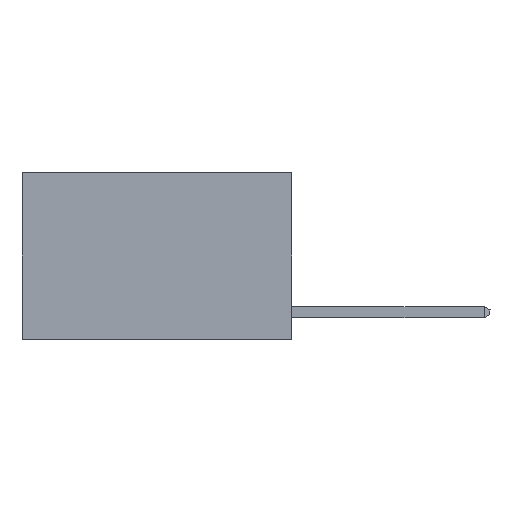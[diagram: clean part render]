
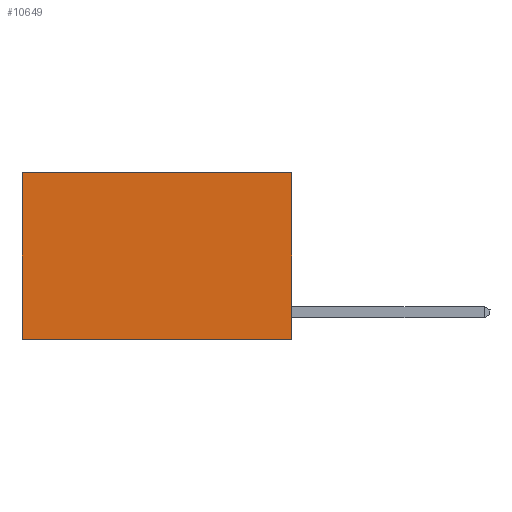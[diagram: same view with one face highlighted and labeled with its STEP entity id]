
A CAD part, left-side view. The second image highlights one B-rep face of the part: STEP entity #10649.
In plain terms, the highlighted planar face has unit normal (-1, 0, 0).
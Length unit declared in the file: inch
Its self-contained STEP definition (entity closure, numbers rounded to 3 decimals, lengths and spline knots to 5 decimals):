
#182 = VERTEX_POINT ( 'NONE', #7796 ) ;
#1017 = VERTEX_POINT ( 'NONE', #14099 ) ;
#1336 = DIRECTION ( 'NONE',  ( 0., 0., -1. ) ) ;
#1639 = VERTEX_POINT ( 'NONE', #2881 ) ;
#1961 = AXIS2_PLACEMENT_3D ( 'NONE', #16460, #17045, #13552 ) ;
#2840 = VERTEX_POINT ( 'NONE', #18826 ) ;
#2881 = CARTESIAN_POINT ( 'NONE',  ( 0.2625, 0., 0. ) ) ;
#3463 = DIRECTION ( 'NONE',  ( 0., 1., 0. ) ) ;
#4207 = CARTESIAN_POINT ( 'NONE',  ( 0.2625, 0.6, 0. ) ) ;
#4495 = DIRECTION ( 'NONE',  ( 0., 0., -1. ) ) ;
#4700 = VECTOR ( 'NONE', #20944, 39.37008 ) ;
#4824 = ORIENTED_EDGE ( 'NONE', *, *, #8897, .F. ) ;
#4926 = VECTOR ( 'NONE', #1336, 39.37008 ) ;
#5048 = EDGE_CURVE ( 'NONE', #182, #2840, #18545, .T. ) ;
#7713 = VECTOR ( 'NONE', #4495, 39.37008 ) ;
#7796 = CARTESIAN_POINT ( 'NONE',  ( 0.2625, 0.6, 0. ) ) ;
#7850 = LINE ( 'NONE', #14981, #4926 ) ;
#8897 = EDGE_CURVE ( 'NONE', #1639, #1017, #7850, .T. ) ;
#10649 = ADVANCED_FACE ( 'NONE', ( #10968 ), #14754, .F. ) ;
#10968 = FACE_OUTER_BOUND ( 'NONE', #13861, .T. ) ;
#12573 = CARTESIAN_POINT ( 'NONE',  ( 0.2625, 0., 0. ) ) ;
#12874 = ORIENTED_EDGE ( 'NONE', *, *, #18933, .F. ) ;
#13237 = EDGE_CURVE ( 'NONE', #1639, #182, #20606, .T. ) ;
#13552 = DIRECTION ( 'NONE',  ( 0., 0., -1. ) ) ;
#13861 = EDGE_LOOP ( 'NONE', ( #16590, #12874, #4824, #19040 ) ) ;
#14099 = CARTESIAN_POINT ( 'NONE',  ( 0.2625, 0., -0.37 ) ) ;
#14754 = PLANE ( 'NONE',  #1961 ) ;
#14981 = CARTESIAN_POINT ( 'NONE',  ( 0.2625, 0., 0. ) ) ;
#16460 = CARTESIAN_POINT ( 'NONE',  ( 0.2625, 0., 0. ) ) ;
#16590 = ORIENTED_EDGE ( 'NONE', *, *, #5048, .T. ) ;
#17045 = DIRECTION ( 'NONE',  ( 1., 0., 0. ) ) ;
#18545 = LINE ( 'NONE', #4207, #7713 ) ;
#18826 = CARTESIAN_POINT ( 'NONE',  ( 0.2625, 0.6, -0.37 ) ) ;
#18933 = EDGE_CURVE ( 'NONE', #1017, #2840, #21726, .T. ) ;
#19040 = ORIENTED_EDGE ( 'NONE', *, *, #13237, .T. ) ;
#19627 = VECTOR ( 'NONE', #3463, 39.37008 ) ;
#20488 = CARTESIAN_POINT ( 'NONE',  ( 0.2625, 0., -0.37 ) ) ;
#20606 = LINE ( 'NONE', #12573, #4700 ) ;
#20944 = DIRECTION ( 'NONE',  ( 0., 1., 0. ) ) ;
#21726 = LINE ( 'NONE', #20488, #19627 ) ;
